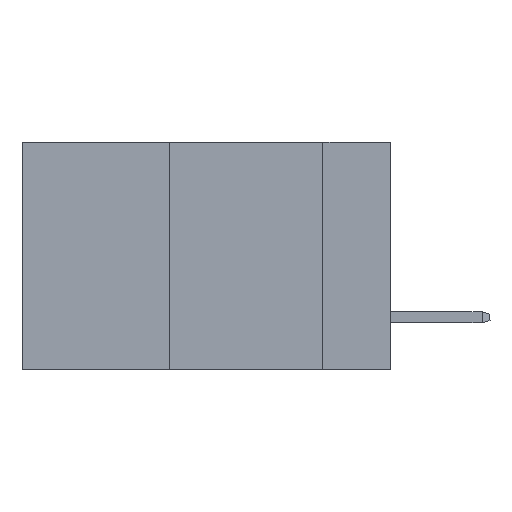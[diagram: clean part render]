
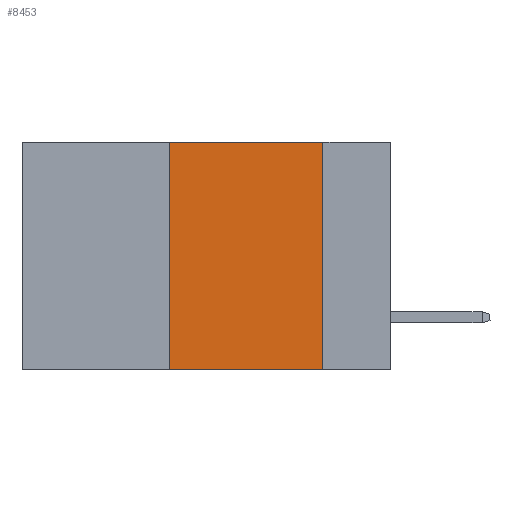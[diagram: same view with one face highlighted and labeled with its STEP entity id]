
A CAD part, left-side view. The second image highlights one B-rep face of the part: STEP entity #8453.
In plain terms, the highlighted planar face has unit normal (-1, 0, 0).
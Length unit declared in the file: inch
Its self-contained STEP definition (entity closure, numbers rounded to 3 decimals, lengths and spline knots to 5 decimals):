
#121 = PLANE ( 'NONE',  #1337 ) ;
#274 = EDGE_CURVE ( 'NONE', #6789, #773, #6243, .T. ) ;
#773 = VERTEX_POINT ( 'NONE', #4968 ) ;
#1074 = DIRECTION ( 'NONE',  ( 0., 0., -1. ) ) ;
#1337 = AXIS2_PLACEMENT_3D ( 'NONE', #3930, #6820, #1074 ) ;
#1407 = CARTESIAN_POINT ( 'NONE',  ( 0., 0.11, 0. ) ) ;
#1931 = ORIENTED_EDGE ( 'NONE', *, *, #8124, .T. ) ;
#2096 = LINE ( 'NONE', #1407, #9465 ) ;
#2282 = VECTOR ( 'NONE', #2630, 39.37008 ) ;
#2630 = DIRECTION ( 'NONE',  ( 0., -1., 0. ) ) ;
#3907 = FACE_OUTER_BOUND ( 'NONE', #9778, .T. ) ;
#3930 = CARTESIAN_POINT ( 'NONE',  ( 0., 0.6, 0. ) ) ;
#4638 = LINE ( 'NONE', #12093, #12317 ) ;
#4769 = ORIENTED_EDGE ( 'NONE', *, *, #274, .F. ) ;
#4968 = CARTESIAN_POINT ( 'NONE',  ( 0., 0.36, 0. ) ) ;
#5514 = CARTESIAN_POINT ( 'NONE',  ( 0., 0.36, -0.37 ) ) ;
#6031 = EDGE_CURVE ( 'NONE', #773, #7685, #7979, .T. ) ;
#6243 = LINE ( 'NONE', #6829, #8495 ) ;
#6789 = VERTEX_POINT ( 'NONE', #5514 ) ;
#6820 = DIRECTION ( 'NONE',  ( 1., 0., 0. ) ) ;
#6829 = CARTESIAN_POINT ( 'NONE',  ( 0., 0.36, 0. ) ) ;
#6912 = ORIENTED_EDGE ( 'NONE', *, *, #7416, .F. ) ;
#7195 = VERTEX_POINT ( 'NONE', #11869 ) ;
#7416 = EDGE_CURVE ( 'NONE', #7685, #7195, #2096, .T. ) ;
#7685 = VERTEX_POINT ( 'NONE', #10492 ) ;
#7979 = LINE ( 'NONE', #8354, #2282 ) ;
#8111 = DIRECTION ( 'NONE',  ( 0., 0., -1. ) ) ;
#8124 = EDGE_CURVE ( 'NONE', #6789, #7195, #4638, .T. ) ;
#8354 = CARTESIAN_POINT ( 'NONE',  ( 0., 0.6, 0. ) ) ;
#8453 = ADVANCED_FACE ( 'NONE', ( #3907 ), #121, .F. ) ;
#8495 = VECTOR ( 'NONE', #10786, 39.37008 ) ;
#9243 = DIRECTION ( 'NONE',  ( 0., -1., 0. ) ) ;
#9465 = VECTOR ( 'NONE', #8111, 39.37008 ) ;
#9778 = EDGE_LOOP ( 'NONE', ( #6912, #10493, #4769, #1931 ) ) ;
#10492 = CARTESIAN_POINT ( 'NONE',  ( 0., 0.11, 0. ) ) ;
#10493 = ORIENTED_EDGE ( 'NONE', *, *, #6031, .F. ) ;
#10786 = DIRECTION ( 'NONE',  ( 0., 0., 1. ) ) ;
#11869 = CARTESIAN_POINT ( 'NONE',  ( 0., 0.11, -0.37 ) ) ;
#12093 = CARTESIAN_POINT ( 'NONE',  ( 0., 0.6, -0.37 ) ) ;
#12317 = VECTOR ( 'NONE', #9243, 39.37008 ) ;
